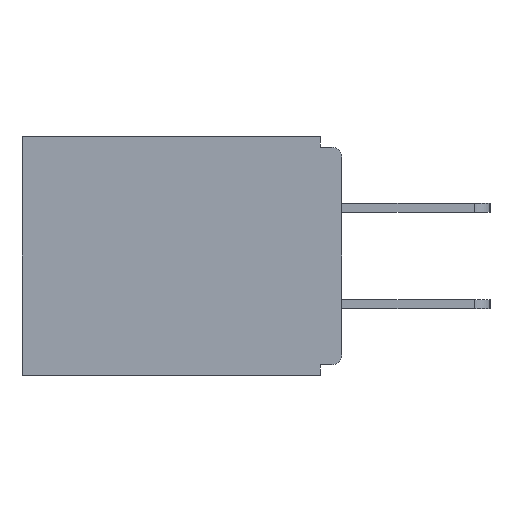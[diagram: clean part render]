
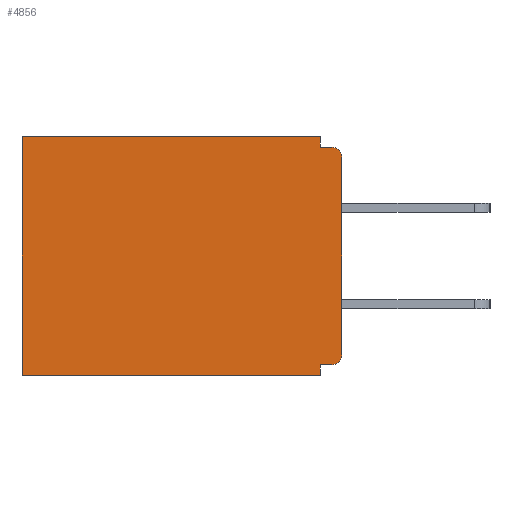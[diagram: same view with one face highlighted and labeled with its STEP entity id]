
A CAD part, left-side view. The second image highlights one B-rep face of the part: STEP entity #4856.
In plain terms, the highlighted planar face has unit normal (-1, 0, 0).
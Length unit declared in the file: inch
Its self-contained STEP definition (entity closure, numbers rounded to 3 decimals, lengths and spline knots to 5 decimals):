
#57 = DIRECTION ( 'NONE',  ( 0., 1., 0. ) ) ;
#512 = VECTOR ( 'NONE', #8783, 39.37008 ) ;
#582 = CARTESIAN_POINT ( 'NONE',  ( 0.298, 0., 0. ) ) ;
#675 = EDGE_CURVE ( 'NONE', #11800, #1208, #5859, .T. ) ;
#887 = EDGE_CURVE ( 'NONE', #1208, #6559, #4749, .T. ) ;
#1208 = VERTEX_POINT ( 'NONE', #12537 ) ;
#1350 = CARTESIAN_POINT ( 'NONE',  ( 0.298, 0.015, -0.313 ) ) ;
#1566 = EDGE_CURVE ( 'NONE', #13426, #3350, #5813, .T. ) ;
#1628 = CARTESIAN_POINT ( 'NONE',  ( 0.298, 0.46, 0. ) ) ;
#1736 = DIRECTION ( 'NONE',  ( 0., 0., -1. ) ) ;
#1771 = CARTESIAN_POINT ( 'NONE',  ( 0.298, 0.015, -0.328 ) ) ;
#1787 = CARTESIAN_POINT ( 'NONE',  ( 0.298, 0., -0.313 ) ) ;
#2213 = DIRECTION ( 'NONE',  ( 0., 0., -1. ) ) ;
#2412 = CARTESIAN_POINT ( 'NONE',  ( 0.298, 0., -0.015 ) ) ;
#2663 = EDGE_CURVE ( 'NONE', #4621, #6559, #11187, .T. ) ;
#2731 = VECTOR ( 'NONE', #10623, 39.37008 ) ;
#2984 = CARTESIAN_POINT ( 'NONE',  ( 0.298, 0.031, -0.343 ) ) ;
#3109 = LINE ( 'NONE', #2412, #2731 ) ;
#3350 = VERTEX_POINT ( 'NONE', #1787 ) ;
#3689 = VECTOR ( 'NONE', #6217, 39.37008 ) ;
#3782 = VECTOR ( 'NONE', #12201, 39.37008 ) ;
#3926 = ORIENTED_EDGE ( 'NONE', *, *, #8456, .T. ) ;
#4428 = AXIS2_PLACEMENT_3D ( 'NONE', #8160, #6913, #2213 ) ;
#4621 = VERTEX_POINT ( 'NONE', #2984 ) ;
#4687 = AXIS2_PLACEMENT_3D ( 'NONE', #12628, #13805, #8855 ) ;
#4748 = AXIS2_PLACEMENT_3D ( 'NONE', #1350, #14425, #11949 ) ;
#4749 = LINE ( 'NONE', #1628, #11053 ) ;
#4799 = ORIENTED_EDGE ( 'NONE', *, *, #1566, .T. ) ;
#4856 = ADVANCED_FACE ( 'NONE', ( #9852 ), #5537, .F. ) ;
#5361 = DIRECTION ( 'NONE',  ( 0., 0., -1. ) ) ;
#5537 = PLANE ( 'NONE',  #4687 ) ;
#5813 = CIRCLE ( 'NONE', #4748, 0.015 ) ;
#5859 = LINE ( 'NONE', #13016, #9002 ) ;
#6217 = DIRECTION ( 'NONE',  ( 0., 0., -1. ) ) ;
#6374 = LINE ( 'NONE', #582, #512 ) ;
#6559 = VERTEX_POINT ( 'NONE', #12785 ) ;
#6865 = EDGE_CURVE ( 'NONE', #11800, #12032, #12418, .T. ) ;
#6913 = DIRECTION ( 'NONE',  ( -1., 0., 0. ) ) ;
#7136 = ORIENTED_EDGE ( 'NONE', *, *, #675, .T. ) ;
#7168 = ORIENTED_EDGE ( 'NONE', *, *, #6865, .F. ) ;
#7212 = ORIENTED_EDGE ( 'NONE', *, *, #14628, .F. ) ;
#7396 = CARTESIAN_POINT ( 'NONE',  ( 0.298, 0.031, -0.343 ) ) ;
#7466 = CARTESIAN_POINT ( 'NONE',  ( 0.298, 0.031, -0.328 ) ) ;
#7540 = CARTESIAN_POINT ( 'NONE',  ( 0.298, 0.031, -0.015 ) ) ;
#7671 = ORIENTED_EDGE ( 'NONE', *, *, #887, .T. ) ;
#7819 = VECTOR ( 'NONE', #1736, 39.37008 ) ;
#8160 = CARTESIAN_POINT ( 'NONE',  ( 0.298, 0.015, -0.03 ) ) ;
#8456 = EDGE_CURVE ( 'NONE', #9106, #12839, #10122, .T. ) ;
#8477 = CARTESIAN_POINT ( 'NONE',  ( 0.298, 0., -0.328 ) ) ;
#8505 = EDGE_CURVE ( 'NONE', #12032, #12839, #3109, .T. ) ;
#8783 = DIRECTION ( 'NONE',  ( 0., 0., -1. ) ) ;
#8855 = DIRECTION ( 'NONE',  ( 0., 0., -1. ) ) ;
#9002 = VECTOR ( 'NONE', #57, 39.37008 ) ;
#9106 = VERTEX_POINT ( 'NONE', #14447 ) ;
#9292 = CARTESIAN_POINT ( 'NONE',  ( 0.298, 0.015, -0.015 ) ) ;
#9340 = LINE ( 'NONE', #11178, #7819 ) ;
#9561 = ORIENTED_EDGE ( 'NONE', *, *, #15076, .F. ) ;
#9654 = CARTESIAN_POINT ( 'NONE',  ( 0.298, 0.031, 0. ) ) ;
#9727 = EDGE_LOOP ( 'NONE', ( #3926, #10988, #7168, #7136, #7671, #14005, #9561, #10693, #4799, #7212 ) ) ;
#9750 = CARTESIAN_POINT ( 'NONE',  ( 0.298, 0., -0.343 ) ) ;
#9852 = FACE_OUTER_BOUND ( 'NONE', #9727, .T. ) ;
#10122 = CIRCLE ( 'NONE', #4428, 0.015 ) ;
#10623 = DIRECTION ( 'NONE',  ( 0., -1., 0. ) ) ;
#10693 = ORIENTED_EDGE ( 'NONE', *, *, #11472, .F. ) ;
#10789 = DIRECTION ( 'NONE',  ( 0., 1., 0. ) ) ;
#10961 = LINE ( 'NONE', #8477, #13005 ) ;
#10988 = ORIENTED_EDGE ( 'NONE', *, *, #8505, .F. ) ;
#11053 = VECTOR ( 'NONE', #5361, 39.37008 ) ;
#11178 = CARTESIAN_POINT ( 'NONE',  ( 0.298, 0.031, -0.343 ) ) ;
#11187 = LINE ( 'NONE', #9750, #3782 ) ;
#11472 = EDGE_CURVE ( 'NONE', #13426, #15169, #10961, .T. ) ;
#11800 = VERTEX_POINT ( 'NONE', #9654 ) ;
#11949 = DIRECTION ( 'NONE',  ( 0., 0., -1. ) ) ;
#12032 = VERTEX_POINT ( 'NONE', #7540 ) ;
#12201 = DIRECTION ( 'NONE',  ( 0., 1., 0. ) ) ;
#12418 = LINE ( 'NONE', #7396, #3689 ) ;
#12537 = CARTESIAN_POINT ( 'NONE',  ( 0.298, 0.46, 0. ) ) ;
#12628 = CARTESIAN_POINT ( 'NONE',  ( 0.298, 0., 0. ) ) ;
#12785 = CARTESIAN_POINT ( 'NONE',  ( 0.298, 0.46, -0.343 ) ) ;
#12839 = VERTEX_POINT ( 'NONE', #9292 ) ;
#13005 = VECTOR ( 'NONE', #10789, 39.37008 ) ;
#13016 = CARTESIAN_POINT ( 'NONE',  ( 0.298, 0., 0. ) ) ;
#13426 = VERTEX_POINT ( 'NONE', #1771 ) ;
#13805 = DIRECTION ( 'NONE',  ( 1., 0., 0. ) ) ;
#14005 = ORIENTED_EDGE ( 'NONE', *, *, #2663, .F. ) ;
#14425 = DIRECTION ( 'NONE',  ( -1., 0., 0. ) ) ;
#14447 = CARTESIAN_POINT ( 'NONE',  ( 0.298, 0., -0.03 ) ) ;
#14628 = EDGE_CURVE ( 'NONE', #9106, #3350, #6374, .T. ) ;
#15076 = EDGE_CURVE ( 'NONE', #15169, #4621, #9340, .T. ) ;
#15169 = VERTEX_POINT ( 'NONE', #7466 ) ;
